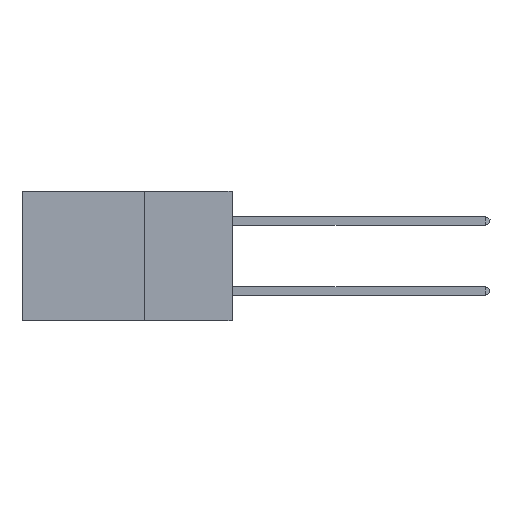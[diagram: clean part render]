
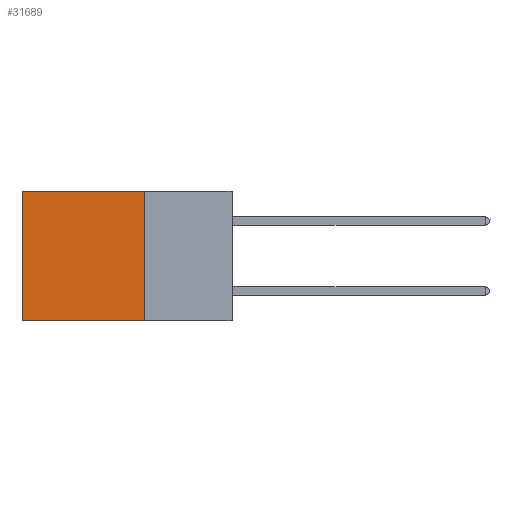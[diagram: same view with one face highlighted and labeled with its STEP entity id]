
A CAD part, left-side view. The second image highlights one B-rep face of the part: STEP entity #31689.
In plain terms, the highlighted planar face has unit normal (-1, 0, 0).
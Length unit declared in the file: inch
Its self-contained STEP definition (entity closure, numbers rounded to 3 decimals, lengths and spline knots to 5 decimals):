
#736 = VERTEX_POINT ( 'NONE', #42797 ) ;
#1474 = AXIS2_PLACEMENT_3D ( 'NONE', #21607, #47407, #21941 ) ;
#3022 = LINE ( 'NONE', #30296, #10529 ) ;
#6979 = VECTOR ( 'NONE', #24171, 39.37008 ) ;
#7319 = VERTEX_POINT ( 'NONE', #19930 ) ;
#9633 = ORIENTED_EDGE ( 'NONE', *, *, #38049, .T. ) ;
#10529 = VECTOR ( 'NONE', #15805, 39.37008 ) ;
#12815 = EDGE_LOOP ( 'NONE', ( #38957, #39063, #28994, #9633 ) ) ;
#12955 = LINE ( 'NONE', #30608, #15278 ) ;
#14100 = PLANE ( 'NONE',  #1474 ) ;
#15278 = VECTOR ( 'NONE', #22779, 39.37008 ) ;
#15805 = DIRECTION ( 'NONE',  ( 0., 0., -1. ) ) ;
#17078 = CARTESIAN_POINT ( 'NONE',  ( 0.2875, 0.25, 0. ) ) ;
#18103 = CARTESIAN_POINT ( 'NONE',  ( 0.2875, 0.6, 0. ) ) ;
#19930 = CARTESIAN_POINT ( 'NONE',  ( 0.2875, 0.25, -0.37 ) ) ;
#21607 = CARTESIAN_POINT ( 'NONE',  ( 0.2875, 0.25, 0. ) ) ;
#21941 = DIRECTION ( 'NONE',  ( 0., 0., -1. ) ) ;
#22221 = CARTESIAN_POINT ( 'NONE',  ( 0.2875, 0.25, 0. ) ) ;
#22779 = DIRECTION ( 'NONE',  ( 0., 1., 0. ) ) ;
#24171 = DIRECTION ( 'NONE',  ( 0., 0., -1. ) ) ;
#25993 = DIRECTION ( 'NONE',  ( 0., 1., 0. ) ) ;
#28380 = LINE ( 'NONE', #22221, #33061 ) ;
#28994 = ORIENTED_EDGE ( 'NONE', *, *, #47163, .F. ) ;
#30296 = CARTESIAN_POINT ( 'NONE',  ( 0.2875, 0.6, 0. ) ) ;
#30608 = CARTESIAN_POINT ( 'NONE',  ( 0.2875, 0.25, -0.37 ) ) ;
#31689 = ADVANCED_FACE ( 'NONE', ( #48184 ), #14100, .F. ) ;
#33061 = VECTOR ( 'NONE', #25993, 39.37008 ) ;
#33520 = VERTEX_POINT ( 'NONE', #47926 ) ;
#38049 = EDGE_CURVE ( 'NONE', #33520, #48041, #28380, .T. ) ;
#38926 = EDGE_CURVE ( 'NONE', #48041, #736, #3022, .T. ) ;
#38957 = ORIENTED_EDGE ( 'NONE', *, *, #38926, .T. ) ;
#39063 = ORIENTED_EDGE ( 'NONE', *, *, #44913, .F. ) ;
#42797 = CARTESIAN_POINT ( 'NONE',  ( 0.2875, 0.6, -0.37 ) ) ;
#44303 = LINE ( 'NONE', #17078, #6979 ) ;
#44913 = EDGE_CURVE ( 'NONE', #7319, #736, #12955, .T. ) ;
#47163 = EDGE_CURVE ( 'NONE', #33520, #7319, #44303, .T. ) ;
#47407 = DIRECTION ( 'NONE',  ( 1., 0., 0. ) ) ;
#47926 = CARTESIAN_POINT ( 'NONE',  ( 0.2875, 0.25, 0. ) ) ;
#48041 = VERTEX_POINT ( 'NONE', #18103 ) ;
#48184 = FACE_OUTER_BOUND ( 'NONE', #12815, .T. ) ;
